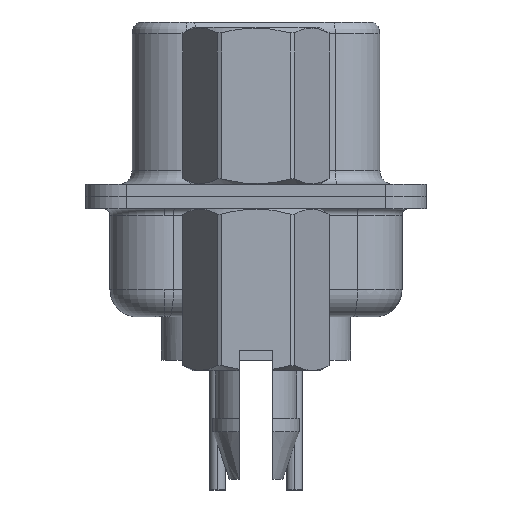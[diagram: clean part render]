
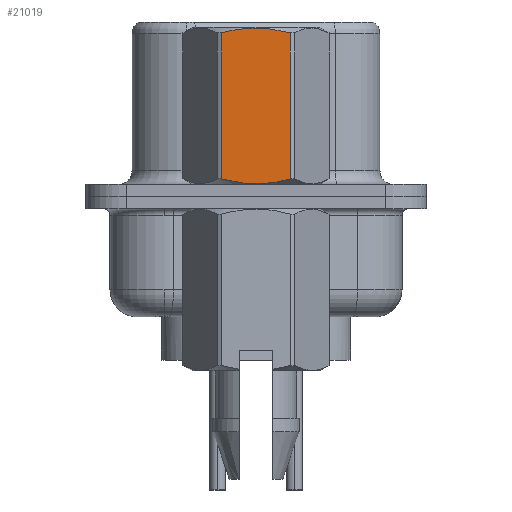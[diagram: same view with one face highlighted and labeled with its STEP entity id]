
A CAD part, left-side view. The second image highlights one B-rep face of the part: STEP entity #21019.
In plain terms, the highlighted planar face has unit normal (-1, 0, 0).
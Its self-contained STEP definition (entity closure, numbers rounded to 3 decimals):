
#326 = ORIENTED_EDGE ( 'NONE', *, *, #25560, .T. ) ;
#1405 = CARTESIAN_POINT ( 'NONE',  ( -2.381, -1.066, 0.596 ) ) ;
#1766 = VECTOR ( 'NONE', #26022, 1000. ) ;
#1992 = CARTESIAN_POINT ( 'NONE',  ( -2.381, 1.273, 6.048 ) ) ;
#2213 = LINE ( 'NONE', #23056, #17560 ) ;
#2378 = CARTESIAN_POINT ( 'NONE',  ( -2.381, -0.432, 6.215 ) ) ;
#3498 = CARTESIAN_POINT ( 'NONE',  ( -2.381, -0.215, 0.468 ) ) ;
#3945 = ORIENTED_EDGE ( 'NONE', *, *, #23038, .T. ) ;
#3992 = VERTEX_POINT ( 'NONE', #14770 ) ;
#5282 = B_SPLINE_CURVE_WITH_KNOTS ( 'NONE', 3,
 ( #27236, #15050, #10384, #2378, #10518, #25173, #12855, #27100, #10919, #23092 ),
 .UNSPECIFIED., .F., .F.,
 ( 4, 2, 2, 2, 4 ),
 ( 0.001, 0.002, 0.002, 0.003, 0.004 ),
 .UNSPECIFIED. ) ;
#5687 = CARTESIAN_POINT ( 'NONE',  ( -2.381, -0.858, 0.55 ) ) ;
#6255 = DIRECTION ( 'NONE',  ( -1., 0., 0. ) ) ;
#6513 = DIRECTION ( 'NONE',  ( 0., -1., 0. ) ) ;
#7926 = EDGE_LOOP ( 'NONE', ( #8185, #3945, #20089, #326 ) ) ;
#8185 = ORIENTED_EDGE ( 'NONE', *, *, #18291, .T. ) ;
#8393 = VERTEX_POINT ( 'NONE', #1992 ) ;
#9685 = CARTESIAN_POINT ( 'NONE',  ( -2.381, -0.432, 0.485 ) ) ;
#10384 = CARTESIAN_POINT ( 'NONE',  ( -2.381, -0.858, 6.15 ) ) ;
#10518 = CARTESIAN_POINT ( 'NONE',  ( -2.381, -0.215, 6.232 ) ) ;
#10618 = DIRECTION ( 'NONE',  ( 0., 0., 1. ) ) ;
#10919 = CARTESIAN_POINT ( 'NONE',  ( -2.381, 1.065, 6.104 ) ) ;
#12439 = FACE_OUTER_BOUND ( 'NONE', #7926, .T. ) ;
#12855 = CARTESIAN_POINT ( 'NONE',  ( -2.381, 0.428, 6.215 ) ) ;
#14100 = CARTESIAN_POINT ( 'NONE',  ( -2.381, -1.273, 0.652 ) ) ;
#14770 = CARTESIAN_POINT ( 'NONE',  ( -2.381, -1.273, 6.048 ) ) ;
#14918 = CARTESIAN_POINT ( 'NONE',  ( -2.381, 1.375, -3.75 ) ) ;
#15050 = CARTESIAN_POINT ( 'NONE',  ( -2.381, -1.066, 6.104 ) ) ;
#15894 = CARTESIAN_POINT ( 'NONE',  ( -2.381, 0.428, 0.485 ) ) ;
#16056 = CARTESIAN_POINT ( 'NONE',  ( -2.381, -1.273, 0.652 ) ) ;
#17560 = VECTOR ( 'NONE', #10618, 1000. ) ;
#18291 = EDGE_CURVE ( 'NONE', #26036, #26482, #26633, .T. ) ;
#19392 = LINE ( 'NONE', #21457, #1766 ) ;
#20089 = ORIENTED_EDGE ( 'NONE', *, *, #20981, .T. ) ;
#20308 = CARTESIAN_POINT ( 'NONE',  ( -2.381, 1.065, 0.596 ) ) ;
#20591 = AXIS2_PLACEMENT_3D ( 'NONE', #14918, #6255, #6513 ) ;
#20981 = EDGE_CURVE ( 'NONE', #3992, #8393, #5282, .T. ) ;
#21019 = ADVANCED_FACE ( 'NONE', ( #12439 ), #25303, .T. ) ;
#21457 = CARTESIAN_POINT ( 'NONE',  ( -2.381, 1.273, 3.792 ) ) ;
#22663 = CARTESIAN_POINT ( 'NONE',  ( -2.381, 0.215, 0.468 ) ) ;
#23038 = EDGE_CURVE ( 'NONE', #26482, #3992, #2213, .T. ) ;
#23056 = CARTESIAN_POINT ( 'NONE',  ( -2.381, -1.273, 3.792 ) ) ;
#23092 = CARTESIAN_POINT ( 'NONE',  ( -2.381, 1.273, 6.048 ) ) ;
#25173 = CARTESIAN_POINT ( 'NONE',  ( -2.381, 0.215, 6.232 ) ) ;
#25303 = PLANE ( 'NONE',  #20591 ) ;
#25560 = EDGE_CURVE ( 'NONE', #8393, #26036, #19392, .T. ) ;
#26022 = DIRECTION ( 'NONE',  ( 0., 0., -1. ) ) ;
#26036 = VERTEX_POINT ( 'NONE', #26918 ) ;
#26482 = VERTEX_POINT ( 'NONE', #16056 ) ;
#26633 = B_SPLINE_CURVE_WITH_KNOTS ( 'NONE', 3,
 ( #26675, #20308, #26952, #15894, #22663, #3498, #9685, #5687, #1405, #14100 ),
 .UNSPECIFIED., .F., .F.,
 ( 4, 2, 2, 2, 4 ),
 ( 0.003, 0.003, 0.004, 0.004, 0.005 ),
 .UNSPECIFIED. ) ;
#26675 = CARTESIAN_POINT ( 'NONE',  ( -2.381, 1.273, 0.652 ) ) ;
#26918 = CARTESIAN_POINT ( 'NONE',  ( -2.381, 1.273, 0.652 ) ) ;
#26952 = CARTESIAN_POINT ( 'NONE',  ( -2.381, 0.853, 0.549 ) ) ;
#27100 = CARTESIAN_POINT ( 'NONE',  ( -2.381, 0.853, 6.151 ) ) ;
#27236 = CARTESIAN_POINT ( 'NONE',  ( -2.381, -1.273, 6.048 ) ) ;
